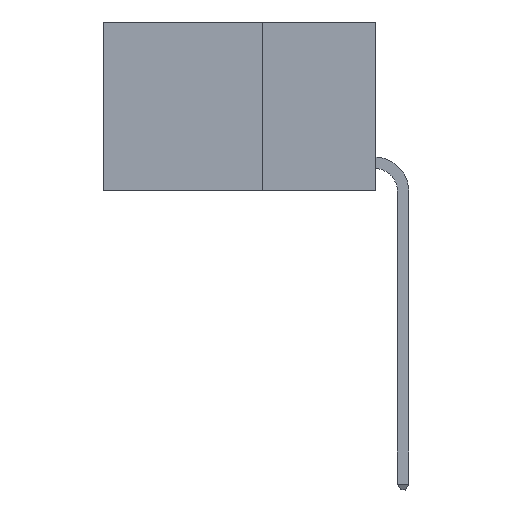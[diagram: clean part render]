
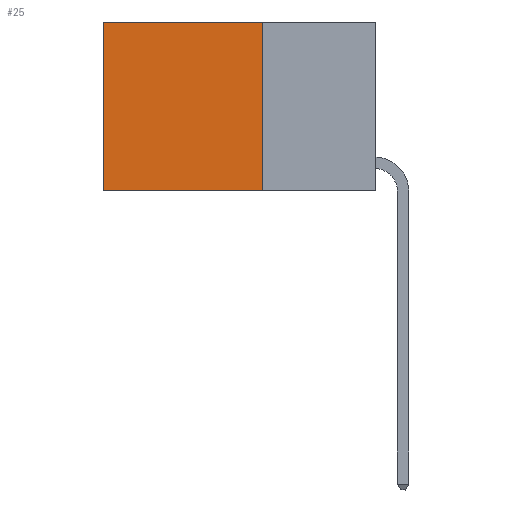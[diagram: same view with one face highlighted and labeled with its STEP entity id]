
A CAD part, left-side view. The second image highlights one B-rep face of the part: STEP entity #25.
In plain terms, the highlighted planar face has unit normal (-1, 0, 0).
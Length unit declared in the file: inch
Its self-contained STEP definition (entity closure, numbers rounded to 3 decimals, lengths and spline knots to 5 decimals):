
#25 = ADVANCED_FACE ( 'NONE', ( #1024 ), #3122, .F. ) ;
#280 = AXIS2_PLACEMENT_3D ( 'NONE', #10060, #12192, #6156 ) ;
#447 = DIRECTION ( 'NONE',  ( 0., 1., 0. ) ) ;
#475 = CARTESIAN_POINT ( 'NONE',  ( 0.2625, 0.25, 0. ) ) ;
#487 = CARTESIAN_POINT ( 'NONE',  ( 0.2625, 0.25, -0.37 ) ) ;
#1024 = FACE_OUTER_BOUND ( 'NONE', #12632, .T. ) ;
#1524 = ORIENTED_EDGE ( 'NONE', *, *, #7840, .T. ) ;
#2257 = LINE ( 'NONE', #487, #7619 ) ;
#2433 = EDGE_CURVE ( 'NONE', #8277, #11114, #6011, .T. ) ;
#2698 = CARTESIAN_POINT ( 'NONE',  ( 0.2625, 0.25, 0. ) ) ;
#3122 = PLANE ( 'NONE',  #280 ) ;
#3733 = DIRECTION ( 'NONE',  ( 0., 0., -1. ) ) ;
#4025 = DIRECTION ( 'NONE',  ( 0., 0., -1. ) ) ;
#4789 = LINE ( 'NONE', #12567, #12212 ) ;
#5323 = VECTOR ( 'NONE', #3733, 39.37008 ) ;
#5695 = VECTOR ( 'NONE', #4025, 39.37008 ) ;
#5955 = LINE ( 'NONE', #2698, #5323 ) ;
#6011 = LINE ( 'NONE', #9040, #5695 ) ;
#6156 = DIRECTION ( 'NONE',  ( 0., 0., -1. ) ) ;
#7201 = VERTEX_POINT ( 'NONE', #475 ) ;
#7619 = VECTOR ( 'NONE', #447, 39.37008 ) ;
#7840 = EDGE_CURVE ( 'NONE', #7201, #8277, #4789, .T. ) ;
#8277 = VERTEX_POINT ( 'NONE', #10244 ) ;
#8477 = EDGE_CURVE ( 'NONE', #9132, #11114, #2257, .T. ) ;
#8763 = ORIENTED_EDGE ( 'NONE', *, *, #8477, .F. ) ;
#9040 = CARTESIAN_POINT ( 'NONE',  ( 0.2625, 0.6, 0. ) ) ;
#9132 = VERTEX_POINT ( 'NONE', #12782 ) ;
#9191 = ORIENTED_EDGE ( 'NONE', *, *, #2433, .T. ) ;
#9272 = ORIENTED_EDGE ( 'NONE', *, *, #12364, .F. ) ;
#9363 = CARTESIAN_POINT ( 'NONE',  ( 0.2625, 0.6, -0.37 ) ) ;
#9501 = DIRECTION ( 'NONE',  ( 0., 1., 0. ) ) ;
#10060 = CARTESIAN_POINT ( 'NONE',  ( 0.2625, 0.25, 0. ) ) ;
#10244 = CARTESIAN_POINT ( 'NONE',  ( 0.2625, 0.6, 0. ) ) ;
#11114 = VERTEX_POINT ( 'NONE', #9363 ) ;
#12192 = DIRECTION ( 'NONE',  ( 1., 0., 0. ) ) ;
#12212 = VECTOR ( 'NONE', #9501, 39.37008 ) ;
#12364 = EDGE_CURVE ( 'NONE', #7201, #9132, #5955, .T. ) ;
#12567 = CARTESIAN_POINT ( 'NONE',  ( 0.2625, 0.25, 0. ) ) ;
#12632 = EDGE_LOOP ( 'NONE', ( #9191, #8763, #9272, #1524 ) ) ;
#12782 = CARTESIAN_POINT ( 'NONE',  ( 0.2625, 0.25, -0.37 ) ) ;
